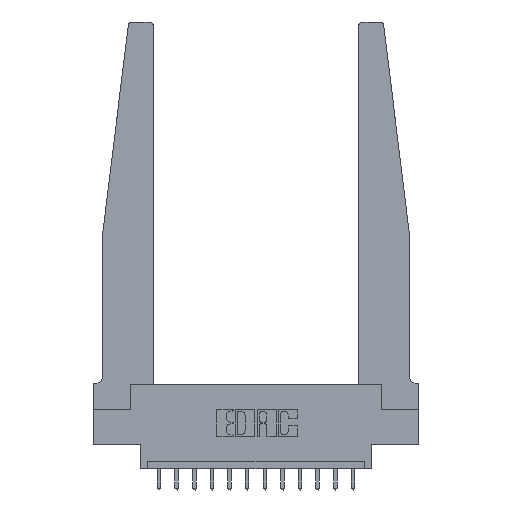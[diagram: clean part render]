
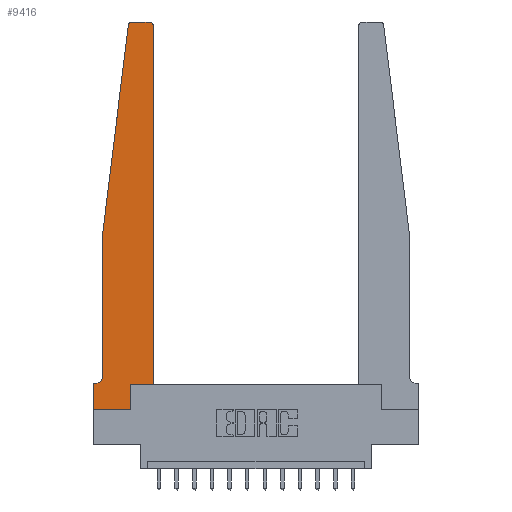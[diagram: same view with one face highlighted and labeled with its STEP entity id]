
A CAD part, top view. The second image highlights one B-rep face of the part: STEP entity #9416.
In plain terms, the highlighted planar face has unit normal (0, 0, 1).
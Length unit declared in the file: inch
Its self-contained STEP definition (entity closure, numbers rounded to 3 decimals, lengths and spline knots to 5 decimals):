
#285 = CARTESIAN_POINT ( 'NONE',  ( 0.015, 0.2375, 0.37 ) ) ;
#562 = VECTOR ( 'NONE', #14561, 39.37008 ) ;
#700 = CARTESIAN_POINT ( 'NONE',  ( 0.065, 1.25, 0.37 ) ) ;
#829 = DIRECTION ( 'NONE',  ( -1., 0., 0. ) ) ;
#836 = LINE ( 'NONE', #13749, #2812 ) ;
#1053 = ORIENTED_EDGE ( 'NONE', *, *, #2093, .T. ) ;
#1414 = LINE ( 'NONE', #10441, #11068 ) ;
#1832 = EDGE_CURVE ( 'NONE', #13842, #13371, #14644, .T. ) ;
#1986 = CARTESIAN_POINT ( 'NONE',  ( 0., 0.1875, 0.37 ) ) ;
#2093 = EDGE_CURVE ( 'NONE', #9561, #11178, #11642, .T. ) ;
#2179 = EDGE_LOOP ( 'NONE', ( #9612, #11551, #6313, #14872, #4332, #1053, #12146, #16044, #4866, #4136, #7302, #7641 ) ) ;
#2355 = CARTESIAN_POINT ( 'NONE',  ( 0.395, 2.72, 0.37 ) ) ;
#2812 = VECTOR ( 'NONE', #14781, 39.37008 ) ;
#3069 = VERTEX_POINT ( 'NONE', #9384 ) ;
#3206 = AXIS2_PLACEMENT_3D ( 'NONE', #6344, #16717, #14154 ) ;
#3251 = PLANE ( 'NONE',  #12737 ) ;
#3343 = VERTEX_POINT ( 'NONE', #6395 ) ;
#3434 = CARTESIAN_POINT ( 'NONE',  ( 0.24675, 2.72367, 0.37 ) ) ;
#3716 = VERTEX_POINT ( 'NONE', #3733 ) ;
#3733 = CARTESIAN_POINT ( 'NONE',  ( 0.2605, 0., 0.37 ) ) ;
#3854 = VECTOR ( 'NONE', #5411, 39.37008 ) ;
#4136 = ORIENTED_EDGE ( 'NONE', *, *, #1832, .T. ) ;
#4221 = LINE ( 'NONE', #13555, #3854 ) ;
#4237 = CARTESIAN_POINT ( 'NONE',  ( 0.425, 0.18, 0.37 ) ) ;
#4300 = CARTESIAN_POINT ( 'NONE',  ( 0.395, 2.75, 0.37 ) ) ;
#4332 = ORIENTED_EDGE ( 'NONE', *, *, #15583, .T. ) ;
#4426 = VECTOR ( 'NONE', #16825, 39.37008 ) ;
#4589 = DIRECTION ( 'NONE',  ( 0., 1., 0. ) ) ;
#4697 = DIRECTION ( 'NONE',  ( 0., -1., 0. ) ) ;
#4866 = ORIENTED_EDGE ( 'NONE', *, *, #10246, .T. ) ;
#5070 = EDGE_CURVE ( 'NONE', #13371, #3069, #836, .T. ) ;
#5265 = CARTESIAN_POINT ( 'NONE',  ( 0.065, 0.1875, 0.37 ) ) ;
#5285 = CARTESIAN_POINT ( 'NONE',  ( 0., 0.1875, 0.37 ) ) ;
#5411 = DIRECTION ( 'NONE',  ( 0., -1., 0. ) ) ;
#5899 = EDGE_CURVE ( 'NONE', #3343, #9235, #10904, .T. ) ;
#6313 = ORIENTED_EDGE ( 'NONE', *, *, #7891, .T. ) ;
#6344 = CARTESIAN_POINT ( 'NONE',  ( 0.27653, 2.72, 0.37 ) ) ;
#6395 = CARTESIAN_POINT ( 'NONE',  ( 0.065, 1.25, 0.37 ) ) ;
#6458 = CIRCLE ( 'NONE', #9183, 0.03 ) ;
#6498 = VECTOR ( 'NONE', #829, 39.37008 ) ;
#6837 = VECTOR ( 'NONE', #9493, 39.37008 ) ;
#7009 = CARTESIAN_POINT ( 'NONE',  ( 0., 0., 0.37 ) ) ;
#7093 = CARTESIAN_POINT ( 'NONE',  ( 0.27653, 2.75, 0.37 ) ) ;
#7120 = LINE ( 'NONE', #16299, #6498 ) ;
#7172 = DIRECTION ( 'NONE',  ( 0., 0., 1. ) ) ;
#7300 = LINE ( 'NONE', #13500, #10850 ) ;
#7302 = ORIENTED_EDGE ( 'NONE', *, *, #5070, .T. ) ;
#7350 = FACE_OUTER_BOUND ( 'NONE', #2179, .T. ) ;
#7641 = ORIENTED_EDGE ( 'NONE', *, *, #8682, .T. ) ;
#7891 = EDGE_CURVE ( 'NONE', #10743, #3343, #1414, .T. ) ;
#7997 = VERTEX_POINT ( 'NONE', #4300 ) ;
#8099 = VERTEX_POINT ( 'NONE', #7093 ) ;
#8321 = LINE ( 'NONE', #7009, #6837 ) ;
#8335 = VECTOR ( 'NONE', #4697, 39.37008 ) ;
#8519 = VERTEX_POINT ( 'NONE', #15078 ) ;
#8682 = EDGE_CURVE ( 'NONE', #3069, #7997, #6458, .T. ) ;
#9037 = CIRCLE ( 'NONE', #9861, 0.05 ) ;
#9076 = DIRECTION ( 'NONE',  ( -0.122, -0.992, 0. ) ) ;
#9183 = AXIS2_PLACEMENT_3D ( 'NONE', #2355, #13926, #11386 ) ;
#9235 = VERTEX_POINT ( 'NONE', #14067 ) ;
#9245 = EDGE_CURVE ( 'NONE', #8099, #10743, #16514, .T. ) ;
#9384 = CARTESIAN_POINT ( 'NONE',  ( 0.425, 2.72, 0.37 ) ) ;
#9416 = ADVANCED_FACE ( 'NONE', ( #7350 ), #3251, .T. ) ;
#9493 = DIRECTION ( 'NONE',  ( 1., 0., 0. ) ) ;
#9561 = VERTEX_POINT ( 'NONE', #10338 ) ;
#9612 = ORIENTED_EDGE ( 'NONE', *, *, #12027, .T. ) ;
#9861 = AXIS2_PLACEMENT_3D ( 'NONE', #285, #14824, #13133 ) ;
#10246 = EDGE_CURVE ( 'NONE', #3716, #13842, #7300, .T. ) ;
#10338 = CARTESIAN_POINT ( 'NONE',  ( 0.015, 0.1875, 0.37 ) ) ;
#10441 = CARTESIAN_POINT ( 'NONE',  ( 0.065, 1.25, 0.37 ) ) ;
#10743 = VERTEX_POINT ( 'NONE', #3434 ) ;
#10850 = VECTOR ( 'NONE', #4589, 39.37008 ) ;
#10904 = LINE ( 'NONE', #700, #8335 ) ;
#11068 = VECTOR ( 'NONE', #9076, 39.37008 ) ;
#11178 = VERTEX_POINT ( 'NONE', #5285 ) ;
#11386 = DIRECTION ( 'NONE',  ( 1., 0., 0. ) ) ;
#11551 = ORIENTED_EDGE ( 'NONE', *, *, #9245, .T. ) ;
#11642 = LINE ( 'NONE', #5265, #4426 ) ;
#12027 = EDGE_CURVE ( 'NONE', #7997, #8099, #7120, .T. ) ;
#12146 = ORIENTED_EDGE ( 'NONE', *, *, #15042, .T. ) ;
#12370 = CARTESIAN_POINT ( 'NONE',  ( 0.2605, 0.18, 0.37 ) ) ;
#12737 = AXIS2_PLACEMENT_3D ( 'NONE', #1986, #7172, #16431 ) ;
#13133 = DIRECTION ( 'NONE',  ( -1., 0., 0. ) ) ;
#13368 = CARTESIAN_POINT ( 'NONE',  ( 0.425, 0.18, 0.37 ) ) ;
#13371 = VERTEX_POINT ( 'NONE', #4237 ) ;
#13500 = CARTESIAN_POINT ( 'NONE',  ( 0.2605, 0.18, 0.37 ) ) ;
#13555 = CARTESIAN_POINT ( 'NONE',  ( 0., 0., 0.37 ) ) ;
#13749 = CARTESIAN_POINT ( 'NONE',  ( 0.425, 0.18, 0.37 ) ) ;
#13842 = VERTEX_POINT ( 'NONE', #12370 ) ;
#13926 = DIRECTION ( 'NONE',  ( 0., 0., 1. ) ) ;
#14067 = CARTESIAN_POINT ( 'NONE',  ( 0.065, 0.2375, 0.37 ) ) ;
#14154 = DIRECTION ( 'NONE',  ( 1., 0., 0. ) ) ;
#14561 = DIRECTION ( 'NONE',  ( 1., 0., 0. ) ) ;
#14644 = LINE ( 'NONE', #13368, #562 ) ;
#14781 = DIRECTION ( 'NONE',  ( 0., 1., 0. ) ) ;
#14824 = DIRECTION ( 'NONE',  ( 0., 0., -1. ) ) ;
#14872 = ORIENTED_EDGE ( 'NONE', *, *, #5899, .T. ) ;
#15007 = EDGE_CURVE ( 'NONE', #8519, #3716, #8321, .T. ) ;
#15042 = EDGE_CURVE ( 'NONE', #11178, #8519, #4221, .T. ) ;
#15078 = CARTESIAN_POINT ( 'NONE',  ( 0., 0., 0.37 ) ) ;
#15583 = EDGE_CURVE ( 'NONE', #9235, #9561, #9037, .T. ) ;
#16044 = ORIENTED_EDGE ( 'NONE', *, *, #15007, .T. ) ;
#16299 = CARTESIAN_POINT ( 'NONE',  ( 0.25, 2.75, 0.37 ) ) ;
#16431 = DIRECTION ( 'NONE',  ( 1., 0., 0. ) ) ;
#16514 = CIRCLE ( 'NONE', #3206, 0.03 ) ;
#16717 = DIRECTION ( 'NONE',  ( 0., 0., 1. ) ) ;
#16825 = DIRECTION ( 'NONE',  ( -1., 0., 0. ) ) ;
